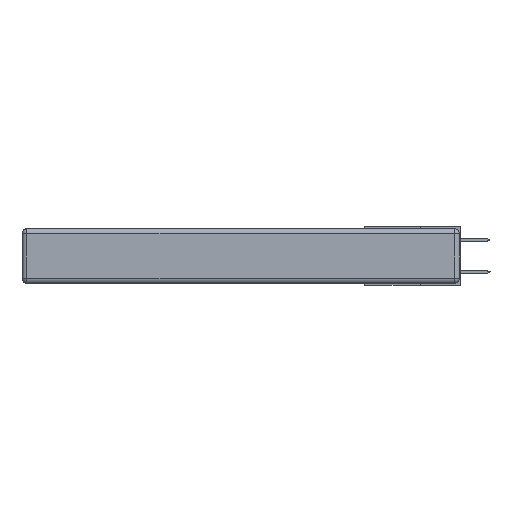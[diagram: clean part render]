
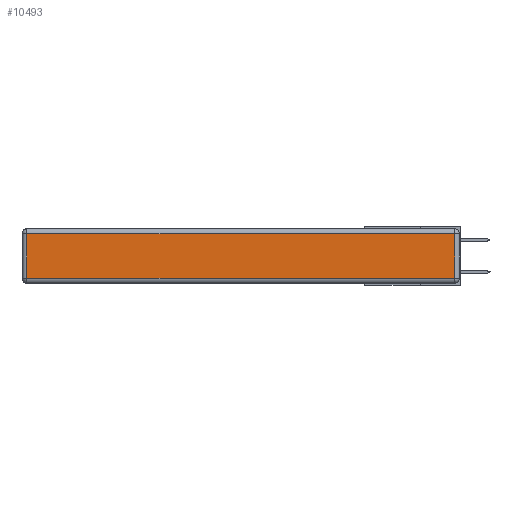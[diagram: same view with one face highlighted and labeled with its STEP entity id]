
A CAD part, left-side view. The second image highlights one B-rep face of the part: STEP entity #10493.
In plain terms, the highlighted planar face has unit normal (-1, 0, 0).
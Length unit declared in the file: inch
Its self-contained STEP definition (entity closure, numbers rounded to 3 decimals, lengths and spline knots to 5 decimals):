
#110 = CARTESIAN_POINT ( 'NONE',  ( 0., 2.75, -0.03 ) ) ;
#1314 = CARTESIAN_POINT ( 'NONE',  ( 0., 0., -0.313 ) ) ;
#1371 = CARTESIAN_POINT ( 'NONE',  ( 0., 2.72, -0.313 ) ) ;
#1437 = EDGE_LOOP ( 'NONE', ( #1718, #3552, #17994, #13886 ) ) ;
#1718 = ORIENTED_EDGE ( 'NONE', *, *, #2728, .T. ) ;
#2111 = VECTOR ( 'NONE', #3920, 39.37008 ) ;
#2454 = LINE ( 'NONE', #1314, #14746 ) ;
#2728 = EDGE_CURVE ( 'NONE', #15393, #17507, #2454, .T. ) ;
#3520 = VERTEX_POINT ( 'NONE', #4598 ) ;
#3552 = ORIENTED_EDGE ( 'NONE', *, *, #14968, .T. ) ;
#3920 = DIRECTION ( 'NONE',  ( 0., 0., 1. ) ) ;
#4013 = PLANE ( 'NONE',  #18184 ) ;
#4598 = CARTESIAN_POINT ( 'NONE',  ( 0., 2.72, -0.03 ) ) ;
#4832 = EDGE_CURVE ( 'NONE', #3520, #15393, #16463, .T. ) ;
#5741 = CARTESIAN_POINT ( 'NONE',  ( 0., 0.03, -0.03 ) ) ;
#5774 = DIRECTION ( 'NONE',  ( 0., 0., 1. ) ) ;
#6549 = EDGE_CURVE ( 'NONE', #13867, #3520, #11820, .T. ) ;
#6831 = CARTESIAN_POINT ( 'NONE',  ( 0., 2.72, -0.343 ) ) ;
#6982 = LINE ( 'NONE', #14867, #2111 ) ;
#7211 = DIRECTION ( 'NONE',  ( -1., 0., 0. ) ) ;
#7600 = CARTESIAN_POINT ( 'NONE',  ( 0., 0.03, -0.313 ) ) ;
#10493 = ADVANCED_FACE ( 'NONE', ( #19966 ), #4013, .T. ) ;
#11820 = LINE ( 'NONE', #110, #18232 ) ;
#13867 = VERTEX_POINT ( 'NONE', #5741 ) ;
#13886 = ORIENTED_EDGE ( 'NONE', *, *, #4832, .T. ) ;
#14746 = VECTOR ( 'NONE', #16061, 39.37008 ) ;
#14867 = CARTESIAN_POINT ( 'NONE',  ( 0., 0.03, -0.343 ) ) ;
#14968 = EDGE_CURVE ( 'NONE', #17507, #13867, #6982, .T. ) ;
#15090 = DIRECTION ( 'NONE',  ( 0., 0., -1. ) ) ;
#15393 = VERTEX_POINT ( 'NONE', #1371 ) ;
#16061 = DIRECTION ( 'NONE',  ( 0., -1., 0. ) ) ;
#16463 = LINE ( 'NONE', #6831, #17019 ) ;
#17019 = VECTOR ( 'NONE', #15090, 39.37008 ) ;
#17507 = VERTEX_POINT ( 'NONE', #7600 ) ;
#17994 = ORIENTED_EDGE ( 'NONE', *, *, #6549, .T. ) ;
#18184 = AXIS2_PLACEMENT_3D ( 'NONE', #18897, #7211, #5774 ) ;
#18232 = VECTOR ( 'NONE', #18851, 39.37008 ) ;
#18851 = DIRECTION ( 'NONE',  ( 0., 1., 0. ) ) ;
#18897 = CARTESIAN_POINT ( 'NONE',  ( 0., 0., -0.343 ) ) ;
#19966 = FACE_OUTER_BOUND ( 'NONE', #1437, .T. ) ;
